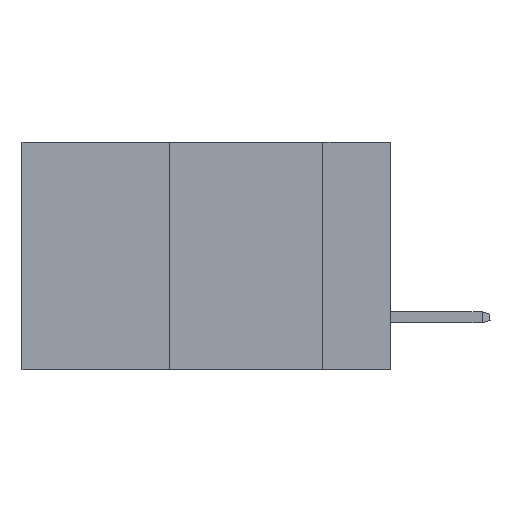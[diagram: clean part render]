
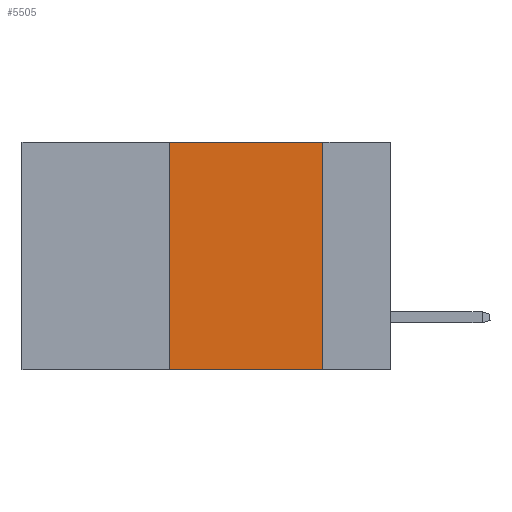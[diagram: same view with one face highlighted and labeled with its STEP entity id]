
A CAD part, left-side view. The second image highlights one B-rep face of the part: STEP entity #5505.
In plain terms, the highlighted planar face has unit normal (-1, 0, 0).
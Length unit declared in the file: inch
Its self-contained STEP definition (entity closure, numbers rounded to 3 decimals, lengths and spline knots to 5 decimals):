
#447 = LINE ( 'NONE', #13559, #22823 ) ;
#1345 = LINE ( 'NONE', #14883, #3699 ) ;
#1696 = DIRECTION ( 'NONE',  ( 0., -1., 0. ) ) ;
#2026 = EDGE_CURVE ( 'NONE', #26154, #15622, #1345, .T. ) ;
#2831 = FACE_OUTER_BOUND ( 'NONE', #27903, .T. ) ;
#3699 = VECTOR ( 'NONE', #23338, 39.37008 ) ;
#5505 = ADVANCED_FACE ( 'NONE', ( #2831 ), #18773, .F. ) ;
#6971 = DIRECTION ( 'NONE',  ( 0., 0., -1. ) ) ;
#7176 = DIRECTION ( 'NONE',  ( 0., 0., 1. ) ) ;
#7454 = VERTEX_POINT ( 'NONE', #16299 ) ;
#7577 = DIRECTION ( 'NONE',  ( 0., -1., 0. ) ) ;
#8511 = ORIENTED_EDGE ( 'NONE', *, *, #25360, .T. ) ;
#8742 = ORIENTED_EDGE ( 'NONE', *, *, #2026, .F. ) ;
#11856 = CARTESIAN_POINT ( 'NONE',  ( 0., 0.6, 0. ) ) ;
#12090 = ORIENTED_EDGE ( 'NONE', *, *, #23133, .F. ) ;
#12744 = CARTESIAN_POINT ( 'NONE',  ( 0., 0.11, -0.37 ) ) ;
#12856 = LINE ( 'NONE', #23281, #13878 ) ;
#13559 = CARTESIAN_POINT ( 'NONE',  ( 0., 0.36, 0. ) ) ;
#13878 = VECTOR ( 'NONE', #1696, 39.37008 ) ;
#14883 = CARTESIAN_POINT ( 'NONE',  ( 0., 0.11, 0. ) ) ;
#14916 = ORIENTED_EDGE ( 'NONE', *, *, #15426, .F. ) ;
#15426 = EDGE_CURVE ( 'NONE', #7454, #26154, #20568, .T. ) ;
#15445 = CARTESIAN_POINT ( 'NONE',  ( 0., 0.11, 0. ) ) ;
#15622 = VERTEX_POINT ( 'NONE', #12744 ) ;
#16299 = CARTESIAN_POINT ( 'NONE',  ( 0., 0.36, 0. ) ) ;
#18773 = PLANE ( 'NONE',  #23097 ) ;
#19148 = DIRECTION ( 'NONE',  ( 1., 0., 0. ) ) ;
#20568 = LINE ( 'NONE', #11856, #25624 ) ;
#22823 = VECTOR ( 'NONE', #7176, 39.37008 ) ;
#23097 = AXIS2_PLACEMENT_3D ( 'NONE', #25593, #19148, #6971 ) ;
#23133 = EDGE_CURVE ( 'NONE', #24504, #7454, #447, .T. ) ;
#23208 = CARTESIAN_POINT ( 'NONE',  ( 0., 0.36, -0.37 ) ) ;
#23281 = CARTESIAN_POINT ( 'NONE',  ( 0., 0.6, -0.37 ) ) ;
#23338 = DIRECTION ( 'NONE',  ( 0., 0., -1. ) ) ;
#24504 = VERTEX_POINT ( 'NONE', #23208 ) ;
#25360 = EDGE_CURVE ( 'NONE', #24504, #15622, #12856, .T. ) ;
#25593 = CARTESIAN_POINT ( 'NONE',  ( 0., 0.6, 0. ) ) ;
#25624 = VECTOR ( 'NONE', #7577, 39.37008 ) ;
#26154 = VERTEX_POINT ( 'NONE', #15445 ) ;
#27903 = EDGE_LOOP ( 'NONE', ( #8742, #14916, #12090, #8511 ) ) ;
